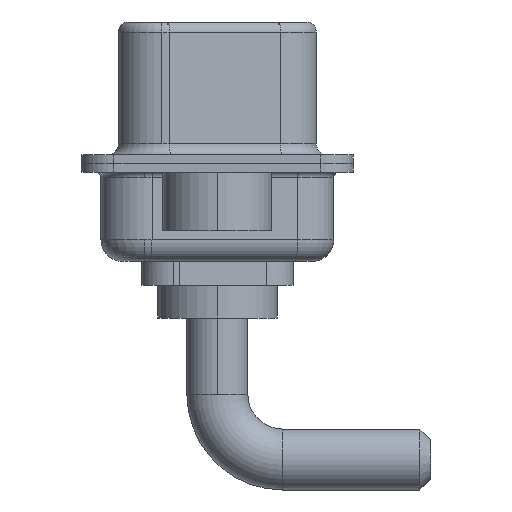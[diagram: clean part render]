
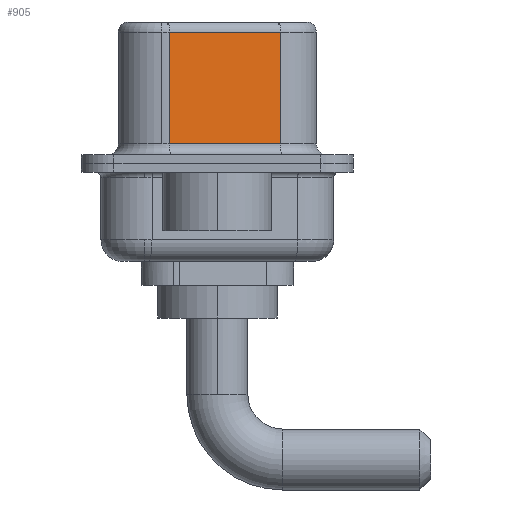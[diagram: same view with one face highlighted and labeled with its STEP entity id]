
A CAD part, left-side view. The second image highlights one B-rep face of the part: STEP entity #905.
In plain terms, the highlighted planar face has unit normal (-0.985, -0.174, 0).
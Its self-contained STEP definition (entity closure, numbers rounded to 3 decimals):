
#2 = ORIENTED_EDGE ( 'NONE', *, *, #7940, .T. ) ;
#341 = CARTESIAN_POINT ( 'NONE',  ( 4.58, -2.897, 6.02 ) ) ;
#539 = EDGE_CURVE ( 'NONE', #9802, #13998, #1114, .T. ) ;
#905 = ADVANCED_FACE ( 'NONE', ( #4363 ), #14142, .F. ) ;
#1114 = LINE ( 'NONE', #3573, #2971 ) ;
#1141 = EDGE_CURVE ( 'NONE', #15434, #13998, #6313, .T. ) ;
#1195 = CARTESIAN_POINT ( 'NONE',  ( 4.58, -2.897, 6.02 ) ) ;
#2971 = VECTOR ( 'NONE', #12130, 1000. ) ;
#2985 = CARTESIAN_POINT ( 'NONE',  ( 4.58, -2.897, 6.52 ) ) ;
#3245 = VECTOR ( 'NONE', #12445, 1000. ) ;
#3558 = LINE ( 'NONE', #7070, #11430 ) ;
#3573 = CARTESIAN_POINT ( 'NONE',  ( 4.58, -2.897, 6.52 ) ) ;
#4363 = FACE_OUTER_BOUND ( 'NONE', #11630, .T. ) ;
#4456 = DIRECTION ( 'NONE',  ( 0., 0., -1. ) ) ;
#5701 = ORIENTED_EDGE ( 'NONE', *, *, #1141, .T. ) ;
#5709 = EDGE_CURVE ( 'NONE', #8161, #15434, #3558, .T. ) ;
#5755 = DIRECTION ( 'NONE',  ( 0.985, 0.174, 0. ) ) ;
#6313 = LINE ( 'NONE', #7538, #9234 ) ;
#7070 = CARTESIAN_POINT ( 'NONE',  ( 3.68, 2.203, 6.52 ) ) ;
#7538 = CARTESIAN_POINT ( 'NONE',  ( 4.58, -2.897, 0.9 ) ) ;
#7940 = EDGE_CURVE ( 'NONE', #9802, #8161, #13991, .T. ) ;
#8161 = VERTEX_POINT ( 'NONE', #14073 ) ;
#8962 = AXIS2_PLACEMENT_3D ( 'NONE', #2985, #5755, #9350 ) ;
#9234 = VECTOR ( 'NONE', #15181, 1000. ) ;
#9350 = DIRECTION ( 'NONE',  ( -0.174, 0.985, 0. ) ) ;
#9802 = VERTEX_POINT ( 'NONE', #341 ) ;
#11118 = ORIENTED_EDGE ( 'NONE', *, *, #5709, .T. ) ;
#11430 = VECTOR ( 'NONE', #4456, 1000. ) ;
#11630 = EDGE_LOOP ( 'NONE', ( #12356, #2, #11118, #5701 ) ) ;
#12130 = DIRECTION ( 'NONE',  ( 0., 0., -1. ) ) ;
#12356 = ORIENTED_EDGE ( 'NONE', *, *, #539, .F. ) ;
#12445 = DIRECTION ( 'NONE',  ( -0.174, 0.985, 0. ) ) ;
#13991 = LINE ( 'NONE', #1195, #3245 ) ;
#13998 = VERTEX_POINT ( 'NONE', #14485 ) ;
#14073 = CARTESIAN_POINT ( 'NONE',  ( 3.68, 2.203, 6.02 ) ) ;
#14142 = PLANE ( 'NONE',  #8962 ) ;
#14485 = CARTESIAN_POINT ( 'NONE',  ( 4.58, -2.897, 0.9 ) ) ;
#14977 = CARTESIAN_POINT ( 'NONE',  ( 3.68, 2.203, 0.9 ) ) ;
#15181 = DIRECTION ( 'NONE',  ( 0.174, -0.985, 0. ) ) ;
#15434 = VERTEX_POINT ( 'NONE', #14977 ) ;
